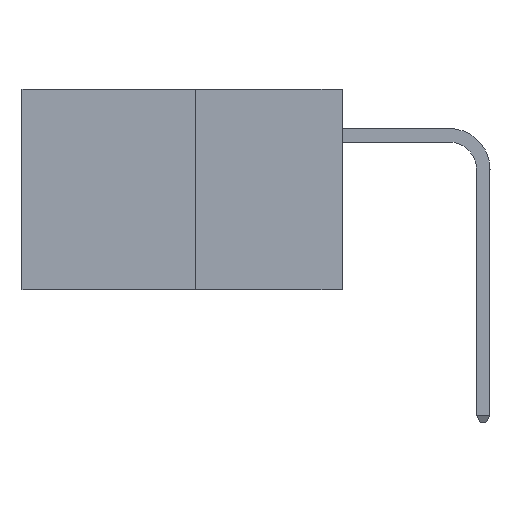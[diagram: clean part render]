
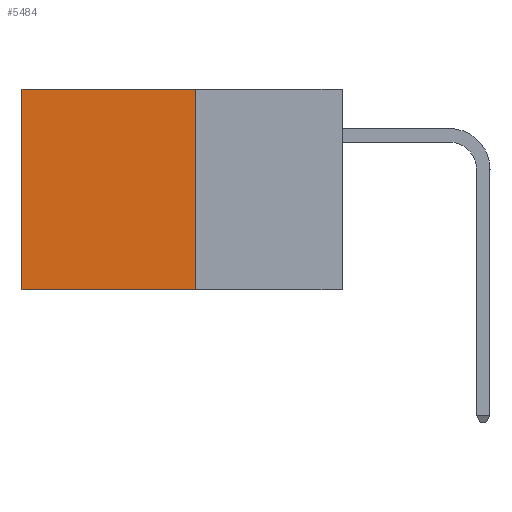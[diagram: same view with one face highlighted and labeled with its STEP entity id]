
A CAD part, left-side view. The second image highlights one B-rep face of the part: STEP entity #5484.
In plain terms, the highlighted planar face has unit normal (-1, 0, 0).
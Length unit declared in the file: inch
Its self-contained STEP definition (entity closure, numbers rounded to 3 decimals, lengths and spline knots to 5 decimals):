
#190 = VERTEX_POINT ( 'NONE', #7247 ) ;
#201 = EDGE_CURVE ( 'NONE', #5581, #190, #2437, .T. ) ;
#437 = AXIS2_PLACEMENT_3D ( 'NONE', #1589, #1587, #1570 ) ;
#569 = CARTESIAN_POINT ( 'NONE',  ( 0.277, 0.27, 0. ) ) ;
#943 = DIRECTION ( 'NONE',  ( 0., 0., -1. ) ) ;
#1570 = DIRECTION ( 'NONE',  ( 0., 0., -1. ) ) ;
#1587 = DIRECTION ( 'NONE',  ( 1., 0., 0. ) ) ;
#1589 = CARTESIAN_POINT ( 'NONE',  ( 0.277, 0.27, -0.37 ) ) ;
#1634 = PLANE ( 'NONE',  #437 ) ;
#2437 = LINE ( 'NONE', #3131, #9677 ) ;
#2566 = VECTOR ( 'NONE', #10789, 39.37008 ) ;
#2913 = EDGE_LOOP ( 'NONE', ( #9605, #9221, #3413, #10176 ) ) ;
#3131 = CARTESIAN_POINT ( 'NONE',  ( 0.277, 0.27, -0.37 ) ) ;
#3413 = ORIENTED_EDGE ( 'NONE', *, *, #201, .F. ) ;
#3807 = EDGE_CURVE ( 'NONE', #10349, #9792, #9780, .T. ) ;
#3930 = EDGE_CURVE ( 'NONE', #5581, #10349, #5075, .T. ) ;
#5075 = LINE ( 'NONE', #10469, #9647 ) ;
#5292 = CARTESIAN_POINT ( 'NONE',  ( 0.277, 0.27, -0.37 ) ) ;
#5484 = ADVANCED_FACE ( 'NONE', ( #6077 ), #1634, .F. ) ;
#5581 = VERTEX_POINT ( 'NONE', #569 ) ;
#6077 = FACE_OUTER_BOUND ( 'NONE', #2913, .T. ) ;
#6125 = CARTESIAN_POINT ( 'NONE',  ( 0.277, 0.59, -0.37 ) ) ;
#7156 = DIRECTION ( 'NONE',  ( 0., 1., 0. ) ) ;
#7173 = VECTOR ( 'NONE', #7156, 39.37008 ) ;
#7247 = CARTESIAN_POINT ( 'NONE',  ( 0.277, 0.27, -0.37 ) ) ;
#7345 = CARTESIAN_POINT ( 'NONE',  ( 0.277, 0.59, 0. ) ) ;
#9221 = ORIENTED_EDGE ( 'NONE', *, *, #10093, .F. ) ;
#9561 = LINE ( 'NONE', #5292, #7173 ) ;
#9605 = ORIENTED_EDGE ( 'NONE', *, *, #3807, .T. ) ;
#9647 = VECTOR ( 'NONE', #10389, 39.37008 ) ;
#9677 = VECTOR ( 'NONE', #943, 39.37008 ) ;
#9780 = LINE ( 'NONE', #6125, #2566 ) ;
#9792 = VERTEX_POINT ( 'NONE', #11301 ) ;
#10093 = EDGE_CURVE ( 'NONE', #190, #9792, #9561, .T. ) ;
#10176 = ORIENTED_EDGE ( 'NONE', *, *, #3930, .T. ) ;
#10349 = VERTEX_POINT ( 'NONE', #7345 ) ;
#10389 = DIRECTION ( 'NONE',  ( 0., 1., 0. ) ) ;
#10469 = CARTESIAN_POINT ( 'NONE',  ( 0.277, 0.27, 0. ) ) ;
#10789 = DIRECTION ( 'NONE',  ( 0., 0., -1. ) ) ;
#11301 = CARTESIAN_POINT ( 'NONE',  ( 0.277, 0.59, -0.37 ) ) ;
